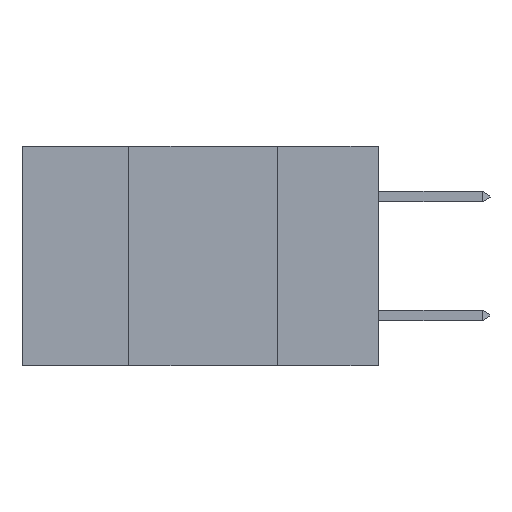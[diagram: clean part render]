
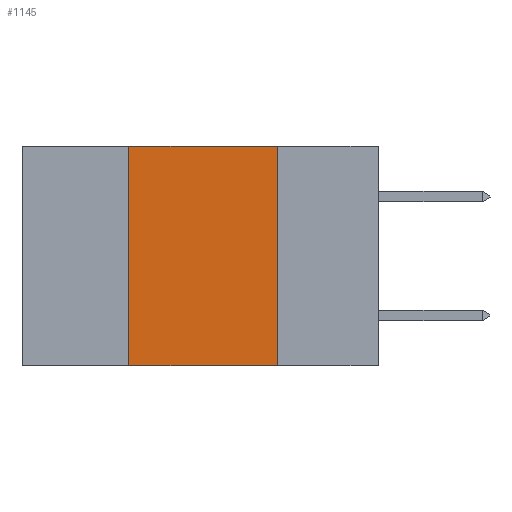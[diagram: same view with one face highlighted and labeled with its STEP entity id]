
A CAD part, left-side view. The second image highlights one B-rep face of the part: STEP entity #1145.
In plain terms, the highlighted planar face has unit normal (-1, 0, 0).
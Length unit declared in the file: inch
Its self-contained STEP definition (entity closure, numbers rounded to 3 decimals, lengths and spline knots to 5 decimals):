
#161 = LINE ( 'NONE', #13848, #9954 ) ;
#1145 = ADVANCED_FACE ( 'NONE', ( #9436 ), #3955, .F. ) ;
#2086 = DIRECTION ( 'NONE',  ( 1., 0., 0. ) ) ;
#2770 = VERTEX_POINT ( 'NONE', #8703 ) ;
#2843 = VERTEX_POINT ( 'NONE', #3536 ) ;
#3381 = VERTEX_POINT ( 'NONE', #11894 ) ;
#3536 = CARTESIAN_POINT ( 'NONE',  ( 0., 0.17, -0.37 ) ) ;
#3570 = CARTESIAN_POINT ( 'NONE',  ( 0., 0.42, 0. ) ) ;
#3789 = EDGE_CURVE ( 'NONE', #3381, #2843, #161, .T. ) ;
#3808 = VECTOR ( 'NONE', #9716, 39.37008 ) ;
#3955 = PLANE ( 'NONE',  #11425 ) ;
#4035 = DIRECTION ( 'NONE',  ( 0., 0., -1. ) ) ;
#5897 = LINE ( 'NONE', #20214, #14864 ) ;
#7421 = ORIENTED_EDGE ( 'NONE', *, *, #9627, .T. ) ;
#7642 = CARTESIAN_POINT ( 'NONE',  ( 0., 0.6, 0. ) ) ;
#8074 = CARTESIAN_POINT ( 'NONE',  ( 0., 0.6, 0. ) ) ;
#8703 = CARTESIAN_POINT ( 'NONE',  ( 0., 0.42, 0. ) ) ;
#9436 = FACE_OUTER_BOUND ( 'NONE', #17856, .T. ) ;
#9627 = EDGE_CURVE ( 'NONE', #17019, #2843, #5897, .T. ) ;
#9716 = DIRECTION ( 'NONE',  ( 0., -1., 0. ) ) ;
#9954 = VECTOR ( 'NONE', #13768, 39.37008 ) ;
#11135 = DIRECTION ( 'NONE',  ( 0., -1., 0. ) ) ;
#11320 = EDGE_CURVE ( 'NONE', #17019, #2770, #21041, .T. ) ;
#11425 = AXIS2_PLACEMENT_3D ( 'NONE', #7642, #2086, #4035 ) ;
#11894 = CARTESIAN_POINT ( 'NONE',  ( 0., 0.17, 0. ) ) ;
#12678 = ORIENTED_EDGE ( 'NONE', *, *, #11320, .F. ) ;
#13768 = DIRECTION ( 'NONE',  ( 0., 0., -1. ) ) ;
#13848 = CARTESIAN_POINT ( 'NONE',  ( 0., 0.17, 0. ) ) ;
#14864 = VECTOR ( 'NONE', #11135, 39.37008 ) ;
#16843 = CARTESIAN_POINT ( 'NONE',  ( 0., 0.42, -0.37 ) ) ;
#17019 = VERTEX_POINT ( 'NONE', #16843 ) ;
#17562 = VECTOR ( 'NONE', #18037, 39.37008 ) ;
#17856 = EDGE_LOOP ( 'NONE', ( #22937, #23392, #12678, #7421 ) ) ;
#18037 = DIRECTION ( 'NONE',  ( 0., 0., 1. ) ) ;
#19356 = EDGE_CURVE ( 'NONE', #2770, #3381, #23121, .T. ) ;
#20214 = CARTESIAN_POINT ( 'NONE',  ( 0., 0.6, -0.37 ) ) ;
#21041 = LINE ( 'NONE', #3570, #17562 ) ;
#22937 = ORIENTED_EDGE ( 'NONE', *, *, #3789, .F. ) ;
#23121 = LINE ( 'NONE', #8074, #3808 ) ;
#23392 = ORIENTED_EDGE ( 'NONE', *, *, #19356, .F. ) ;
